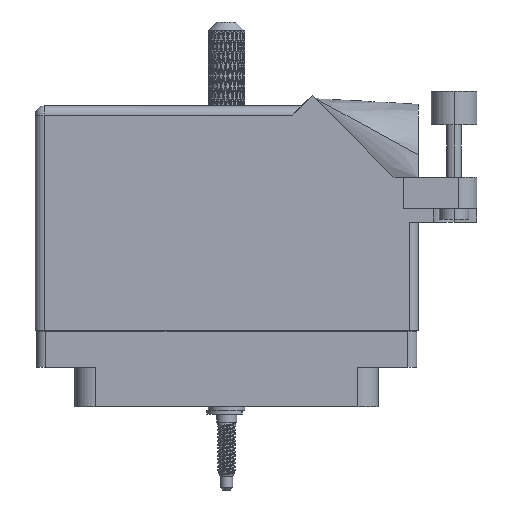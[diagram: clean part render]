
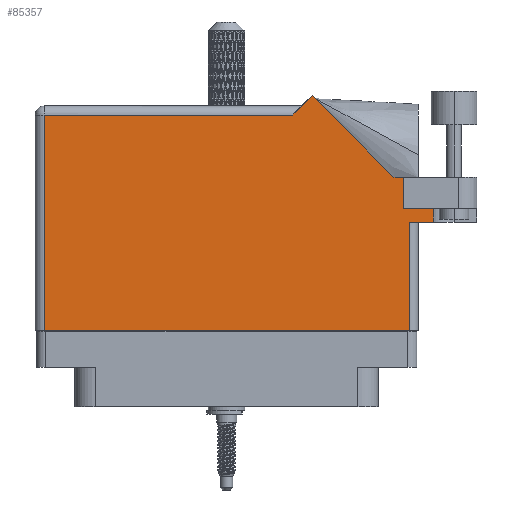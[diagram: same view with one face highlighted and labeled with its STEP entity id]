
A CAD part, front view. The second image highlights one B-rep face of the part: STEP entity #85357.
In plain terms, the highlighted face is planar.
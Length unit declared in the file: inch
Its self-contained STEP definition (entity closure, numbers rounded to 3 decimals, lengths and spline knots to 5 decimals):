
#108 = CARTESIAN_POINT ( 'NONE',  ( 0.451, 1.368, 0.455 ) ) ;
#1244 = DIRECTION ( 'NONE',  ( 1., 0., 0. ) ) ;
#2544 = LINE ( 'NONE', #62831, #23048 ) ;
#2825 = CARTESIAN_POINT ( 'NONE',  ( 1.706, 0.944, 0.455 ) ) ;
#7058 = VERTEX_POINT ( 'NONE', #108 ) ;
#8361 = LINE ( 'NONE', #20690, #57785 ) ;
#9041 = ORIENTED_EDGE ( 'NONE', *, *, #34580, .T. ) ;
#9426 = ORIENTED_EDGE ( 'NONE', *, *, #56186, .T. ) ;
#11640 = VECTOR ( 'NONE', #1244, 39.37008 ) ;
#15099 = ORIENTED_EDGE ( 'NONE', *, *, #25054, .F. ) ;
#15657 = CARTESIAN_POINT ( 'NONE',  ( -1.244, 1.368, 0.455 ) ) ;
#17729 = DIRECTION ( 'NONE',  ( -1., 0., 0. ) ) ;
#18436 = LINE ( 'NONE', #97001, #11640 ) ;
#19989 = EDGE_CURVE ( 'NONE', #66595, #34085, #18436, .T. ) ;
#20690 = CARTESIAN_POINT ( 'NONE',  ( 1.244, 0.637, 0.455 ) ) ;
#21288 = DIRECTION ( 'NONE',  ( 0., 1., 0. ) ) ;
#22768 = CARTESIAN_POINT ( 'NONE',  ( 1.14042, 0.944, 0.455 ) ) ;
#23048 = VECTOR ( 'NONE', #21288, 39.37008 ) ;
#23160 = DIRECTION ( 'NONE',  ( 0., 0., -1. ) ) ;
#23527 = CARTESIAN_POINT ( 'NONE',  ( -1.306, 1.43, 0.455 ) ) ;
#25054 = EDGE_CURVE ( 'NONE', #74137, #60898, #97342, .T. ) ;
#25641 = DIRECTION ( 'NONE',  ( 0., -1., 0. ) ) ;
#25645 = VECTOR ( 'NONE', #25641, 39.37008 ) ;
#27314 = ORIENTED_EDGE ( 'NONE', *, *, #41141, .F. ) ;
#27921 = FACE_OUTER_BOUND ( 'NONE', #36039, .T. ) ;
#29320 = CARTESIAN_POINT ( 'NONE',  ( 1.244, 0.637, 0.455 ) ) ;
#34085 = VERTEX_POINT ( 'NONE', #71910 ) ;
#34227 = DIRECTION ( 'NONE',  ( 1., 0., 0. ) ) ;
#34580 = EDGE_CURVE ( 'NONE', #79027, #85310, #48216, .T. ) ;
#35759 = VECTOR ( 'NONE', #70488, 39.37008 ) ;
#36039 = EDGE_LOOP ( 'NONE', ( #62905, #108174, #46947, #27314, #15099, #107460, #9041, #113589, #9426, #42206, #102347 ) ) ;
#36312 = CARTESIAN_POINT ( 'NONE',  ( 1.206, 0.944, 0.455 ) ) ;
#37971 = DIRECTION ( 'NONE',  ( 0., 1., 0. ) ) ;
#38232 = LINE ( 'NONE', #94987, #67096 ) ;
#38590 = CARTESIAN_POINT ( 'NONE',  ( 0.513, 1.43, 0.455 ) ) ;
#39956 = DIRECTION ( 'NONE',  ( -1., 0., 0. ) ) ;
#41016 = LINE ( 'NONE', #38590, #75421 ) ;
#41141 = EDGE_CURVE ( 'NONE', #60898, #34085, #107926, .T. ) ;
#42206 = ORIENTED_EDGE ( 'NONE', *, *, #66762, .T. ) ;
#46947 = ORIENTED_EDGE ( 'NONE', *, *, #19989, .T. ) ;
#48216 = LINE ( 'NONE', #2825, #81152 ) ;
#48272 = VERTEX_POINT ( 'NONE', #15657 ) ;
#49668 = LINE ( 'NONE', #70258, #93516 ) ;
#50258 = CARTESIAN_POINT ( 'NONE',  ( 1.4075, 1.06177, 0.455 ) ) ;
#54449 = CARTESIAN_POINT ( 'NONE',  ( 1.4075, 0.731, 0.455 ) ) ;
#56186 = EDGE_CURVE ( 'NONE', #82208, #7058, #41016, .T. ) ;
#57785 = VECTOR ( 'NONE', #37971, 39.37008 ) ;
#58741 = AXIS2_PLACEMENT_3D ( 'NONE', #23527, #23160, #101373 ) ;
#59134 = CARTESIAN_POINT ( 'NONE',  ( 1.244, -0.1, 0.455 ) ) ;
#60898 = VERTEX_POINT ( 'NONE', #54449 ) ;
#61022 = CARTESIAN_POINT ( 'NONE',  ( 1.14042, 0.944, 0.455 ) ) ;
#62831 = CARTESIAN_POINT ( 'NONE',  ( 1.206, 0.731, 0.455 ) ) ;
#62905 = ORIENTED_EDGE ( 'NONE', *, *, #79939, .T. ) ;
#66595 = VERTEX_POINT ( 'NONE', #29320 ) ;
#66762 = EDGE_CURVE ( 'NONE', #7058, #48272, #49668, .T. ) ;
#67096 = VECTOR ( 'NONE', #76966, 39.37008 ) ;
#70258 = CARTESIAN_POINT ( 'NONE',  ( -1.306, 1.368, 0.455 ) ) ;
#70488 = DIRECTION ( 'NONE',  ( -0.707, 0.707, 0. ) ) ;
#71487 = DIRECTION ( 'NONE',  ( 0., -1., 0. ) ) ;
#71910 = CARTESIAN_POINT ( 'NONE',  ( 1.4075, 0.637, 0.455 ) ) ;
#74137 = VERTEX_POINT ( 'NONE', #98396 ) ;
#75421 = VECTOR ( 'NONE', #108328, 39.37008 ) ;
#76966 = DIRECTION ( 'NONE',  ( 1., 0., 0. ) ) ;
#79027 = VERTEX_POINT ( 'NONE', #36312 ) ;
#79561 = CARTESIAN_POINT ( 'NONE',  ( -1.244, -0.1, 0.455 ) ) ;
#79939 = EDGE_CURVE ( 'NONE', #87911, #90658, #38232, .T. ) ;
#80376 = VECTOR ( 'NONE', #71487, 39.37008 ) ;
#81152 = VECTOR ( 'NONE', #39956, 39.37008 ) ;
#82208 = VERTEX_POINT ( 'NONE', #92391 ) ;
#82823 = EDGE_CURVE ( 'NONE', #48272, #87911, #87316, .T. ) ;
#85310 = VERTEX_POINT ( 'NONE', #22768 ) ;
#85357 = ADVANCED_FACE ( 'NONE', ( #27921 ), #102132, .F. ) ;
#86454 = VECTOR ( 'NONE', #34227, 39.37008 ) ;
#87316 = LINE ( 'NONE', #79561, #80376 ) ;
#87911 = VERTEX_POINT ( 'NONE', #104773 ) ;
#90658 = VERTEX_POINT ( 'NONE', #59134 ) ;
#92391 = CARTESIAN_POINT ( 'NONE',  ( 0.58371, 1.50071, 0.455 ) ) ;
#93516 = VECTOR ( 'NONE', #17729, 39.37008 ) ;
#94694 = LINE ( 'NONE', #61022, #35759 ) ;
#94987 = CARTESIAN_POINT ( 'NONE',  ( -1.306, -0.1, 0.455 ) ) ;
#95126 = CARTESIAN_POINT ( 'NONE',  ( 1.206, 0.731, 0.455 ) ) ;
#97001 = CARTESIAN_POINT ( 'NONE',  ( 1.306, 0.637, 0.455 ) ) ;
#97342 = LINE ( 'NONE', #95126, #86454 ) ;
#98396 = CARTESIAN_POINT ( 'NONE',  ( 1.206, 0.731, 0.455 ) ) ;
#101373 = DIRECTION ( 'NONE',  ( -1., 0., 0. ) ) ;
#102132 = PLANE ( 'NONE',  #58741 ) ;
#102347 = ORIENTED_EDGE ( 'NONE', *, *, #82823, .T. ) ;
#104773 = CARTESIAN_POINT ( 'NONE',  ( -1.244, -0.1, 0.455 ) ) ;
#105420 = EDGE_CURVE ( 'NONE', #85310, #82208, #94694, .T. ) ;
#107400 = EDGE_CURVE ( 'NONE', #74137, #79027, #2544, .T. ) ;
#107460 = ORIENTED_EDGE ( 'NONE', *, *, #107400, .T. ) ;
#107926 = LINE ( 'NONE', #50258, #25645 ) ;
#108174 = ORIENTED_EDGE ( 'NONE', *, *, #113362, .T. ) ;
#108328 = DIRECTION ( 'NONE',  ( -0.707, -0.707, 0. ) ) ;
#113362 = EDGE_CURVE ( 'NONE', #90658, #66595, #8361, .T. ) ;
#113589 = ORIENTED_EDGE ( 'NONE', *, *, #105420, .T. ) ;
